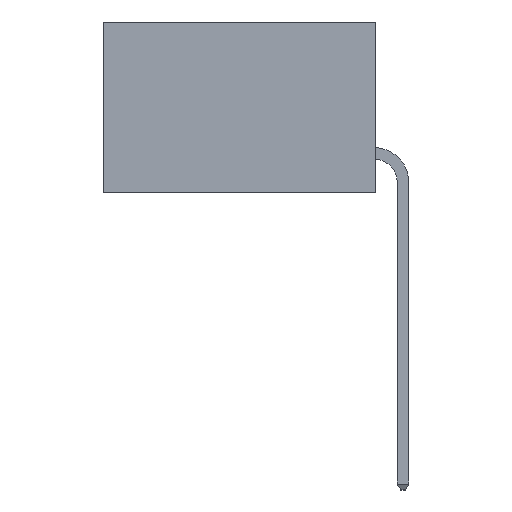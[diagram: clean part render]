
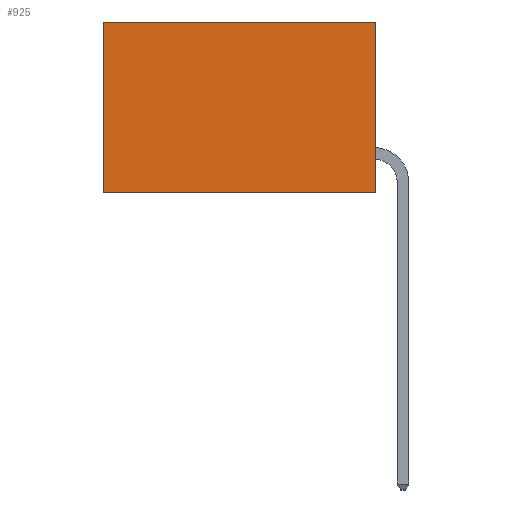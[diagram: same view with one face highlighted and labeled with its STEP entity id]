
A CAD part, left-side view. The second image highlights one B-rep face of the part: STEP entity #925.
In plain terms, the highlighted planar face has unit normal (-1, 0, 0).
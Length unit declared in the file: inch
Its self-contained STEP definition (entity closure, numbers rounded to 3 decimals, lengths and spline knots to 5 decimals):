
#122 = VECTOR ( 'NONE', #5894, 39.37008 ) ;
#171 = EDGE_CURVE ( 'NONE', #3975, #5206, #8447, .T. ) ;
#925 = ADVANCED_FACE ( 'NONE', ( #6082 ), #6089, .F. ) ;
#1159 = ORIENTED_EDGE ( 'NONE', *, *, #5774, .T. ) ;
#1262 = DIRECTION ( 'NONE',  ( 0., 0., -1. ) ) ;
#1281 = ORIENTED_EDGE ( 'NONE', *, *, #171, .F. ) ;
#1347 = ORIENTED_EDGE ( 'NONE', *, *, #3902, .F. ) ;
#1374 = ORIENTED_EDGE ( 'NONE', *, *, #3737, .T. ) ;
#1734 = VECTOR ( 'NONE', #1262, 39.37008 ) ;
#2002 = CARTESIAN_POINT ( 'NONE',  ( 0.277, 0., 0. ) ) ;
#2515 = LINE ( 'NONE', #2918, #122 ) ;
#2684 = CARTESIAN_POINT ( 'NONE',  ( 0.277, 0., -0.37 ) ) ;
#2918 = CARTESIAN_POINT ( 'NONE',  ( 0.277, 0., -0.37 ) ) ;
#3044 = VECTOR ( 'NONE', #8503, 39.37008 ) ;
#3737 = EDGE_CURVE ( 'NONE', #6566, #7300, #6071, .T. ) ;
#3902 = EDGE_CURVE ( 'NONE', #6566, #3975, #2515, .T. ) ;
#3945 = CARTESIAN_POINT ( 'NONE',  ( 0.277, 0.59, -0.37 ) ) ;
#3975 = VERTEX_POINT ( 'NONE', #5598 ) ;
#4299 = DIRECTION ( 'NONE',  ( 1., 0., 0. ) ) ;
#5206 = VERTEX_POINT ( 'NONE', #3945 ) ;
#5377 = CARTESIAN_POINT ( 'NONE',  ( 0.277, 0., -0.37 ) ) ;
#5598 = CARTESIAN_POINT ( 'NONE',  ( 0.277, 0., -0.37 ) ) ;
#5774 = EDGE_CURVE ( 'NONE', #7300, #5206, #9345, .T. ) ;
#5894 = DIRECTION ( 'NONE',  ( 0., 0., -1. ) ) ;
#6071 = LINE ( 'NONE', #9245, #9275 ) ;
#6082 = FACE_OUTER_BOUND ( 'NONE', #6224, .T. ) ;
#6089 = PLANE ( 'NONE',  #7007 ) ;
#6224 = EDGE_LOOP ( 'NONE', ( #1159, #1281, #1347, #1374 ) ) ;
#6566 = VERTEX_POINT ( 'NONE', #2002 ) ;
#6859 = CARTESIAN_POINT ( 'NONE',  ( 0.277, 0.59, 0. ) ) ;
#7007 = AXIS2_PLACEMENT_3D ( 'NONE', #5377, #4299, #9211 ) ;
#7300 = VERTEX_POINT ( 'NONE', #6859 ) ;
#8057 = CARTESIAN_POINT ( 'NONE',  ( 0.277, 0.59, -0.37 ) ) ;
#8447 = LINE ( 'NONE', #2684, #3044 ) ;
#8503 = DIRECTION ( 'NONE',  ( 0., 1., 0. ) ) ;
#9211 = DIRECTION ( 'NONE',  ( 0., 0., -1. ) ) ;
#9245 = CARTESIAN_POINT ( 'NONE',  ( 0.277, 0., 0. ) ) ;
#9258 = DIRECTION ( 'NONE',  ( 0., 1., 0. ) ) ;
#9275 = VECTOR ( 'NONE', #9258, 39.37008 ) ;
#9345 = LINE ( 'NONE', #8057, #1734 ) ;
